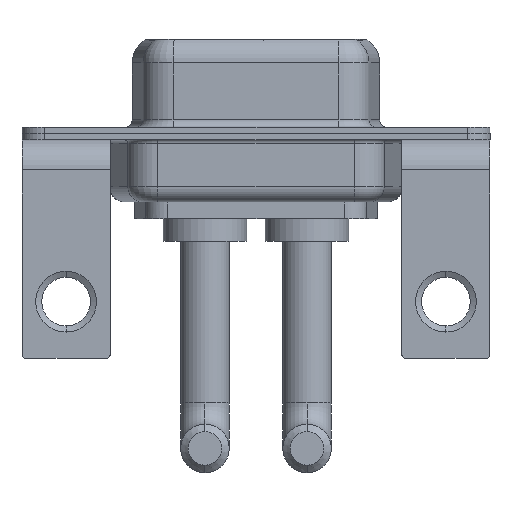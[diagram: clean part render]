
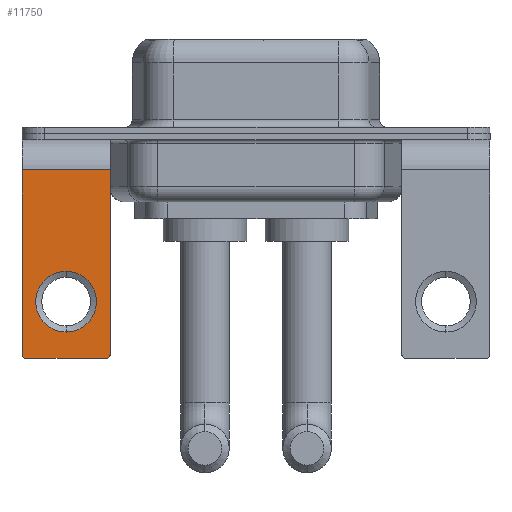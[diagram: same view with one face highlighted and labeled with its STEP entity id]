
A CAD part, front view. The second image highlights one B-rep face of the part: STEP entity #11750.
In plain terms, the highlighted planar face has unit normal (0, -1, 0).
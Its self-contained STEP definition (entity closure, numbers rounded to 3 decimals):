
#135 = CARTESIAN_POINT ( 'NONE',  ( 0., -6.25, -9.07 ) ) ;
#258 = CARTESIAN_POINT ( 'NONE',  ( 0., -6.25, -13.07 ) ) ;
#393 = DIRECTION ( 'NONE',  ( 0., -1., 0. ) ) ;
#595 = CARTESIAN_POINT ( 'NONE',  ( 2.9, -6.25, -2.4 ) ) ;
#739 = CARTESIAN_POINT ( 'NONE',  ( 2.9, -6.25, -2.4 ) ) ;
#741 = PLANE ( 'NONE',  #5236 ) ;
#1067 = DIRECTION ( 'NONE',  ( 0., 0., 1. ) ) ;
#1088 = VERTEX_POINT ( 'NONE', #8517 ) ;
#1584 = CIRCLE ( 'NONE', #5444, 2. ) ;
#2083 = DIRECTION ( 'NONE',  ( 0., 0., -1. ) ) ;
#2336 = CIRCLE ( 'NONE', #9136, 0.25 ) ;
#2434 = EDGE_CURVE ( 'NONE', #10391, #13958, #8648, .T. ) ;
#2634 = DIRECTION ( 'NONE',  ( -1., 0., 0. ) ) ;
#3067 = DIRECTION ( 'NONE',  ( 0., 0., 1. ) ) ;
#3327 = CARTESIAN_POINT ( 'NONE',  ( 2.65, -6.25, -14.8 ) ) ;
#3377 = ORIENTED_EDGE ( 'NONE', *, *, #10448, .T. ) ;
#3731 = DIRECTION ( 'NONE',  ( -1., 0., 0. ) ) ;
#3875 = CARTESIAN_POINT ( 'NONE',  ( 2.9, -6.25, -2.4 ) ) ;
#4156 = LINE ( 'NONE', #5504, #7933 ) ;
#4192 = EDGE_CURVE ( 'NONE', #10391, #12462, #13509, .T. ) ;
#4430 = DIRECTION ( 'NONE',  ( 0., 1., 0. ) ) ;
#4749 = ORIENTED_EDGE ( 'NONE', *, *, #9159, .T. ) ;
#4945 = FACE_BOUND ( 'NONE', #9809, .T. ) ;
#5030 = ORIENTED_EDGE ( 'NONE', *, *, #12655, .T. ) ;
#5122 = DIRECTION ( 'NONE',  ( 0., 1., 0. ) ) ;
#5236 = AXIS2_PLACEMENT_3D ( 'NONE', #3875, #4430, #8639 ) ;
#5376 = EDGE_CURVE ( 'NONE', #10128, #6875, #1584, .T. ) ;
#5444 = AXIS2_PLACEMENT_3D ( 'NONE', #6204, #5122, #3067 ) ;
#5504 = CARTESIAN_POINT ( 'NONE',  ( -2.9, -6.25, -2.4 ) ) ;
#6204 = CARTESIAN_POINT ( 'NONE',  ( 0., -6.25, -11.07 ) ) ;
#6674 = ORIENTED_EDGE ( 'NONE', *, *, #5376, .T. ) ;
#6844 = CIRCLE ( 'NONE', #12102, 2. ) ;
#6875 = VERTEX_POINT ( 'NONE', #135 ) ;
#7540 = CIRCLE ( 'NONE', #8691, 0.25 ) ;
#7581 = VERTEX_POINT ( 'NONE', #12960 ) ;
#7856 = ORIENTED_EDGE ( 'NONE', *, *, #8338, .T. ) ;
#7933 = VECTOR ( 'NONE', #2083, 1000. ) ;
#8116 = VECTOR ( 'NONE', #13014, 1000. ) ;
#8338 = EDGE_CURVE ( 'NONE', #7581, #1088, #2336, .T. ) ;
#8389 = CARTESIAN_POINT ( 'NONE',  ( 2.9, -6.25, -14.8 ) ) ;
#8517 = CARTESIAN_POINT ( 'NONE',  ( -2.65, -6.25, -14.8 ) ) ;
#8639 = DIRECTION ( 'NONE',  ( 0., 0., 1. ) ) ;
#8648 = LINE ( 'NONE', #14058, #8116 ) ;
#8691 = AXIS2_PLACEMENT_3D ( 'NONE', #11926, #11988, #1067 ) ;
#8982 = CARTESIAN_POINT ( 'NONE',  ( -2.9, -6.25, -2.4 ) ) ;
#9136 = AXIS2_PLACEMENT_3D ( 'NONE', #10140, #393, #10072 ) ;
#9159 = EDGE_CURVE ( 'NONE', #11501, #13958, #7540, .T. ) ;
#9232 = ORIENTED_EDGE ( 'NONE', *, *, #4192, .T. ) ;
#9265 = DIRECTION ( 'NONE',  ( 0., 0., 1. ) ) ;
#9437 = EDGE_CURVE ( 'NONE', #11501, #1088, #12423, .T. ) ;
#9809 = EDGE_LOOP ( 'NONE', ( #6674, #5030 ) ) ;
#10072 = DIRECTION ( 'NONE',  ( 0., 0., 1. ) ) ;
#10128 = VERTEX_POINT ( 'NONE', #258 ) ;
#10140 = CARTESIAN_POINT ( 'NONE',  ( -2.65, -6.25, -14.55 ) ) ;
#10391 = VERTEX_POINT ( 'NONE', #739 ) ;
#10448 = EDGE_CURVE ( 'NONE', #12462, #7581, #4156, .T. ) ;
#10466 = DIRECTION ( 'NONE',  ( 0., 1., 0. ) ) ;
#10858 = EDGE_LOOP ( 'NONE', ( #3377, #7856, #11312, #4749, #11756, #9232 ) ) ;
#11312 = ORIENTED_EDGE ( 'NONE', *, *, #9437, .F. ) ;
#11501 = VERTEX_POINT ( 'NONE', #3327 ) ;
#11557 = CARTESIAN_POINT ( 'NONE',  ( 2.9, -6.25, -14.55 ) ) ;
#11750 = ADVANCED_FACE ( 'NONE', ( #4945, #13641 ), #741, .F. ) ;
#11756 = ORIENTED_EDGE ( 'NONE', *, *, #2434, .F. ) ;
#11926 = CARTESIAN_POINT ( 'NONE',  ( 2.65, -6.25, -14.55 ) ) ;
#11988 = DIRECTION ( 'NONE',  ( 0., -1., 0. ) ) ;
#12102 = AXIS2_PLACEMENT_3D ( 'NONE', #12481, #10466, #9265 ) ;
#12423 = LINE ( 'NONE', #8389, #13487 ) ;
#12462 = VERTEX_POINT ( 'NONE', #8982 ) ;
#12481 = CARTESIAN_POINT ( 'NONE',  ( 0., -6.25, -11.07 ) ) ;
#12497 = VECTOR ( 'NONE', #3731, 1000. ) ;
#12655 = EDGE_CURVE ( 'NONE', #6875, #10128, #6844, .T. ) ;
#12960 = CARTESIAN_POINT ( 'NONE',  ( -2.9, -6.25, -14.55 ) ) ;
#13014 = DIRECTION ( 'NONE',  ( 0., 0., -1. ) ) ;
#13487 = VECTOR ( 'NONE', #2634, 1000. ) ;
#13509 = LINE ( 'NONE', #595, #12497 ) ;
#13641 = FACE_OUTER_BOUND ( 'NONE', #10858, .T. ) ;
#13958 = VERTEX_POINT ( 'NONE', #11557 ) ;
#14058 = CARTESIAN_POINT ( 'NONE',  ( 2.9, -6.25, -2.4 ) ) ;
